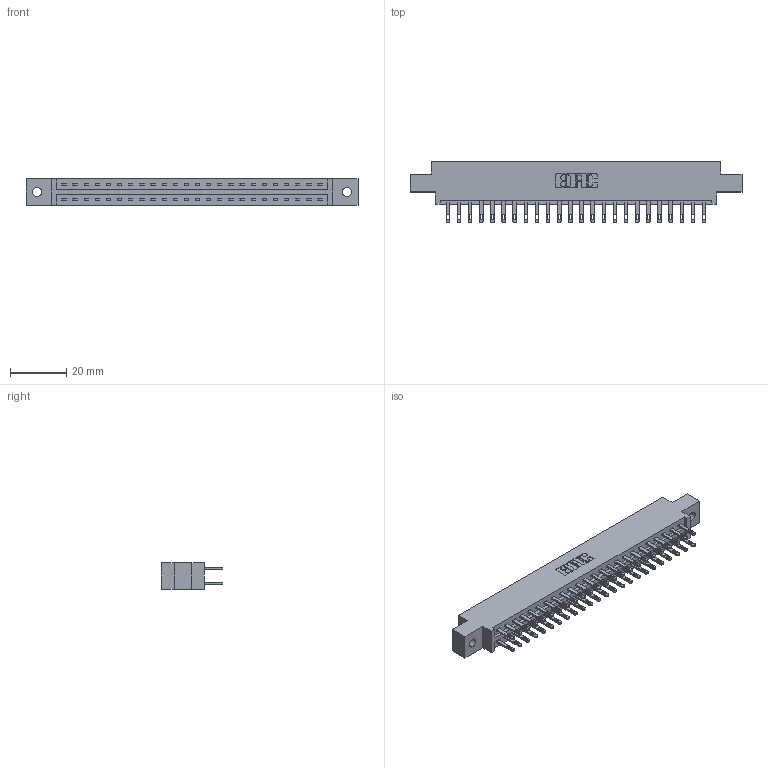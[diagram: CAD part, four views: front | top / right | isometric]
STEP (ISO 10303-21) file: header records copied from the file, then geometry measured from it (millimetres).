
FILE_DESCRIPTION (( 'STEP AP203' ), '1' );
FILE_NAME ('337-048-500-802.STEP', '2019-10-11T15:04:22', ( '' ), ( '' ), 'SwSTEP 2.0', 'SolidWorks 2016', '' );
FILE_SCHEMA (( 'CONFIG_CONTROL_DESIGN' ));
Length unit declared in the file: inch
Products named in the file (3): 337-048-500-802; 337 Part_0.170 Offset - 0.128 Dia; 345-292-001_345-293-100
Assembly tree (49 placements, depth 2):
  337-048-500-802
    337 Part_0.170 Offset - 0.128 Dia
    345-292-001_345-293-100  x48
Bounding box: 118.11 x 21.85 x 9.4 mm (x, y, z)
Volume: 12200.3 mm3; surface area: 13985.3 mm2
Topology: 49 solids, 49 shells, 2518 faces, 7667 edges, 5110 vertices
Faces by surface type: plane 1610, cylinder 908
Entity records: 21001 total; most frequent: CARTESIAN_POINT 3554, ORIENTED_EDGE 3490, DIRECTION 3057, EDGE_CURVE 1745, VECTOR 1613, LINE 1613, VERTEX_POINT 1162, AXIS2_PLACEMENT_3D 722
